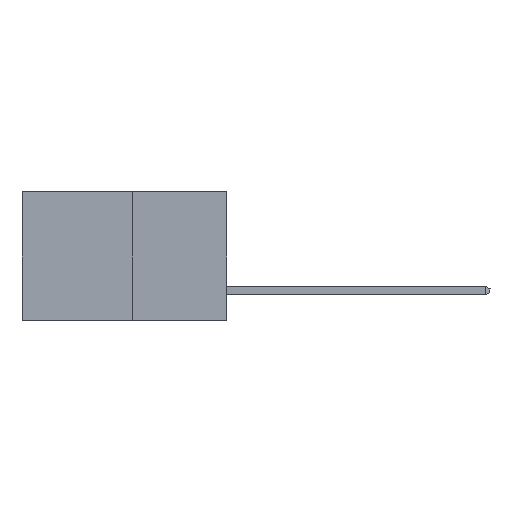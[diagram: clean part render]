
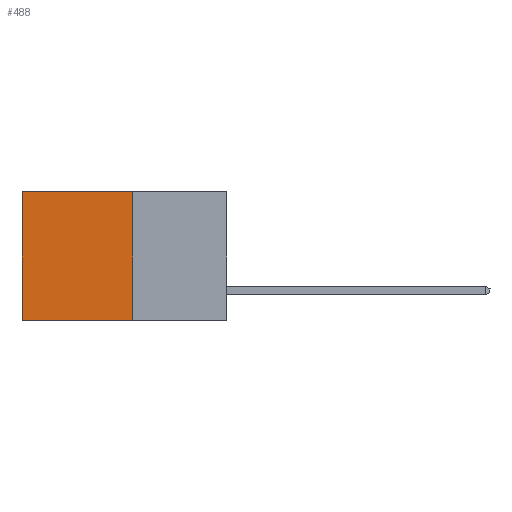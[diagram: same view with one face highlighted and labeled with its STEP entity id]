
A CAD part, left-side view. The second image highlights one B-rep face of the part: STEP entity #488.
In plain terms, the highlighted planar face has unit normal (-1, 0, 0).
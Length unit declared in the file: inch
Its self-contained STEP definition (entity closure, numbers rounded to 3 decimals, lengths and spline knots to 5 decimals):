
#488 = ADVANCED_FACE ( 'NONE', ( #3999 ), #2129, .F. ) ;
#1507 = DIRECTION ( 'NONE',  ( 0., 0., -1. ) ) ;
#1729 = CARTESIAN_POINT ( 'NONE',  ( 0.277, 0.27, 0. ) ) ;
#2129 = PLANE ( 'NONE',  #7122 ) ;
#2703 = VERTEX_POINT ( 'NONE', #8589 ) ;
#2953 = EDGE_CURVE ( 'NONE', #5498, #4518, #8518, .T. ) ;
#3342 = EDGE_CURVE ( 'NONE', #4518, #2703, #11942, .T. ) ;
#3415 = CARTESIAN_POINT ( 'NONE',  ( 0.277, 0.27, -0.37 ) ) ;
#3626 = VECTOR ( 'NONE', #7850, 39.37008 ) ;
#3999 = FACE_OUTER_BOUND ( 'NONE', #10754, .T. ) ;
#4147 = VECTOR ( 'NONE', #9649, 39.37008 ) ;
#4518 = VERTEX_POINT ( 'NONE', #12395 ) ;
#5498 = VERTEX_POINT ( 'NONE', #1729 ) ;
#5792 = CARTESIAN_POINT ( 'NONE',  ( 0.277, 0.27, -0.37 ) ) ;
#6582 = DIRECTION ( 'NONE',  ( 1., 0., 0. ) ) ;
#6648 = ORIENTED_EDGE ( 'NONE', *, *, #13072, .T. ) ;
#6915 = VECTOR ( 'NONE', #1507, 39.37008 ) ;
#7122 = AXIS2_PLACEMENT_3D ( 'NONE', #9125, #6582, #10837 ) ;
#7125 = CARTESIAN_POINT ( 'NONE',  ( 0.277, 0.59, -0.37 ) ) ;
#7850 = DIRECTION ( 'NONE',  ( 0., 1., 0. ) ) ;
#8518 = LINE ( 'NONE', #3415, #10978 ) ;
#8589 = CARTESIAN_POINT ( 'NONE',  ( 0.277, 0.59, -0.37 ) ) ;
#9125 = CARTESIAN_POINT ( 'NONE',  ( 0.277, 0.27, -0.37 ) ) ;
#9310 = DIRECTION ( 'NONE',  ( 0., 0., -1. ) ) ;
#9472 = EDGE_CURVE ( 'NONE', #5498, #11064, #9971, .T. ) ;
#9649 = DIRECTION ( 'NONE',  ( 0., 1., 0. ) ) ;
#9677 = CARTESIAN_POINT ( 'NONE',  ( 0.277, 0.27, 0. ) ) ;
#9971 = LINE ( 'NONE', #9677, #4147 ) ;
#10149 = ORIENTED_EDGE ( 'NONE', *, *, #2953, .F. ) ;
#10754 = EDGE_LOOP ( 'NONE', ( #6648, #13098, #10149, #13755 ) ) ;
#10837 = DIRECTION ( 'NONE',  ( 0., 0., -1. ) ) ;
#10978 = VECTOR ( 'NONE', #9310, 39.37008 ) ;
#11064 = VERTEX_POINT ( 'NONE', #13014 ) ;
#11942 = LINE ( 'NONE', #5792, #3626 ) ;
#12395 = CARTESIAN_POINT ( 'NONE',  ( 0.277, 0.27, -0.37 ) ) ;
#12504 = LINE ( 'NONE', #7125, #6915 ) ;
#13014 = CARTESIAN_POINT ( 'NONE',  ( 0.277, 0.59, 0. ) ) ;
#13072 = EDGE_CURVE ( 'NONE', #11064, #2703, #12504, .T. ) ;
#13098 = ORIENTED_EDGE ( 'NONE', *, *, #3342, .F. ) ;
#13755 = ORIENTED_EDGE ( 'NONE', *, *, #9472, .T. ) ;
